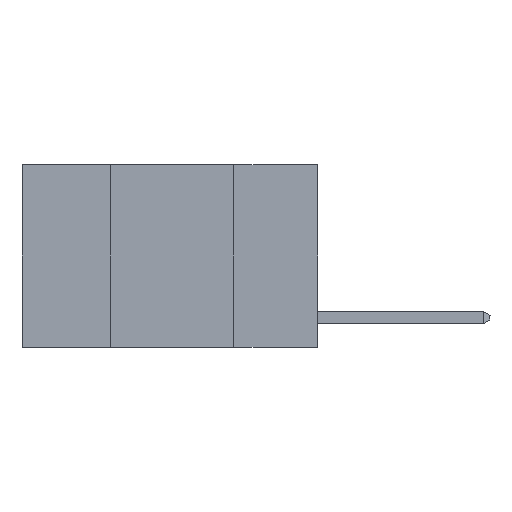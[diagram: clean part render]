
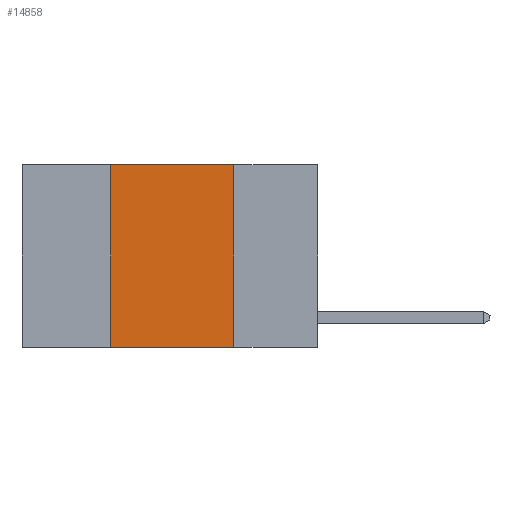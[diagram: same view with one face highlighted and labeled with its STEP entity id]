
A CAD part, left-side view. The second image highlights one B-rep face of the part: STEP entity #14858.
In plain terms, the highlighted planar face has unit normal (-1, 0, 0).
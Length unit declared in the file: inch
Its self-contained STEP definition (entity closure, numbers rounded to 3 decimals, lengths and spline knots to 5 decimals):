
#1381 = CARTESIAN_POINT ( 'NONE',  ( 0., 0.6, -0.37 ) ) ;
#2196 = CARTESIAN_POINT ( 'NONE',  ( 0., 0.42, -0.37 ) ) ;
#3313 = DIRECTION ( 'NONE',  ( 1., 0., 0. ) ) ;
#3771 = PLANE ( 'NONE',  #17007 ) ;
#4456 = CARTESIAN_POINT ( 'NONE',  ( 0., 0.42, 0. ) ) ;
#4623 = CARTESIAN_POINT ( 'NONE',  ( 0., 0.17, -0.37 ) ) ;
#4636 = LINE ( 'NONE', #6441, #8162 ) ;
#6266 = LINE ( 'NONE', #4456, #15112 ) ;
#6441 = CARTESIAN_POINT ( 'NONE',  ( 0., 0.17, 0. ) ) ;
#7919 = DIRECTION ( 'NONE',  ( 0., -1., 0. ) ) ;
#8162 = VECTOR ( 'NONE', #16612, 39.37008 ) ;
#9921 = EDGE_LOOP ( 'NONE', ( #19575, #16807, #13028, #11287 ) ) ;
#10134 = VECTOR ( 'NONE', #7919, 39.37008 ) ;
#10300 = CARTESIAN_POINT ( 'NONE',  ( 0., 0.6, 0. ) ) ;
#11287 = ORIENTED_EDGE ( 'NONE', *, *, #18727, .T. ) ;
#11996 = EDGE_CURVE ( 'NONE', #20389, #16776, #6266, .T. ) ;
#13028 = ORIENTED_EDGE ( 'NONE', *, *, #11996, .F. ) ;
#13078 = DIRECTION ( 'NONE',  ( 0., -1., 0. ) ) ;
#13956 = CARTESIAN_POINT ( 'NONE',  ( 0., 0.42, 0. ) ) ;
#14283 = EDGE_CURVE ( 'NONE', #18843, #18831, #4636, .T. ) ;
#14858 = ADVANCED_FACE ( 'NONE', ( #15042 ), #3771, .F. ) ;
#15042 = FACE_OUTER_BOUND ( 'NONE', #9921, .T. ) ;
#15112 = VECTOR ( 'NONE', #18386, 39.37008 ) ;
#16044 = VECTOR ( 'NONE', #13078, 39.37008 ) ;
#16612 = DIRECTION ( 'NONE',  ( 0., 0., -1. ) ) ;
#16776 = VERTEX_POINT ( 'NONE', #13956 ) ;
#16807 = ORIENTED_EDGE ( 'NONE', *, *, #20996, .F. ) ;
#17007 = AXIS2_PLACEMENT_3D ( 'NONE', #10300, #3313, #21052 ) ;
#18060 = CARTESIAN_POINT ( 'NONE',  ( 0., 0.6, 0. ) ) ;
#18386 = DIRECTION ( 'NONE',  ( 0., 0., 1. ) ) ;
#18399 = LINE ( 'NONE', #18060, #16044 ) ;
#18727 = EDGE_CURVE ( 'NONE', #20389, #18831, #22141, .T. ) ;
#18831 = VERTEX_POINT ( 'NONE', #4623 ) ;
#18843 = VERTEX_POINT ( 'NONE', #22028 ) ;
#19575 = ORIENTED_EDGE ( 'NONE', *, *, #14283, .F. ) ;
#20389 = VERTEX_POINT ( 'NONE', #2196 ) ;
#20996 = EDGE_CURVE ( 'NONE', #16776, #18843, #18399, .T. ) ;
#21052 = DIRECTION ( 'NONE',  ( 0., 0., -1. ) ) ;
#22028 = CARTESIAN_POINT ( 'NONE',  ( 0., 0.17, 0. ) ) ;
#22141 = LINE ( 'NONE', #1381, #10134 ) ;
